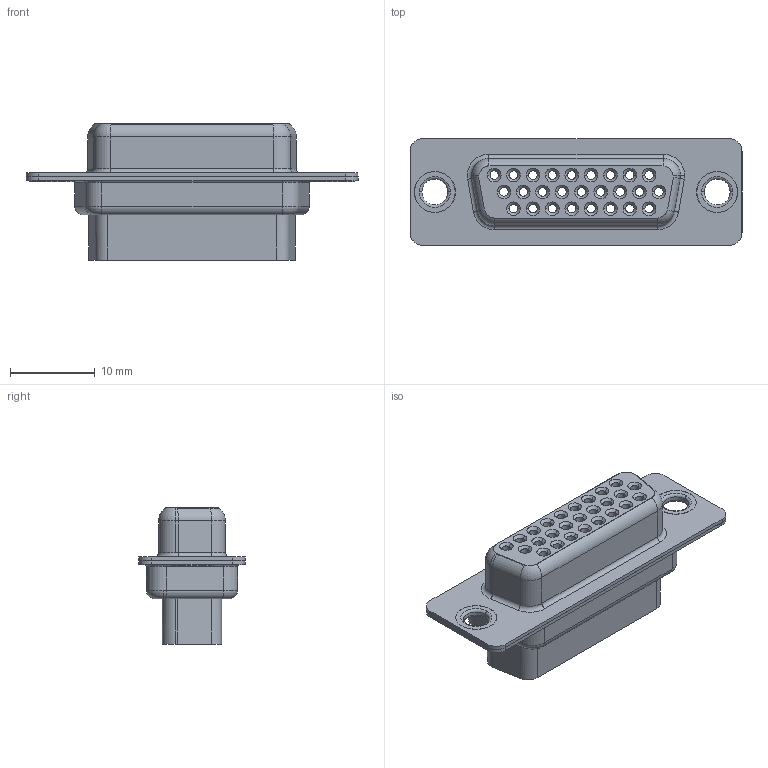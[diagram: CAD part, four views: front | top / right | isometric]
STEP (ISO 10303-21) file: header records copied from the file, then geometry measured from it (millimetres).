
FILE_DESCRIPTION (( 'STEP AP203' ), '1' );
FILE_NAME ('638-026-010-041.STEP', '2020-07-18T16:34:46', ( '' ), ( '' ), 'SwSTEP 2.0', 'SolidWorks 2020', '' );
FILE_SCHEMA (( 'CONFIG_CONTROL_DESIGN' ));
Length unit declared in the file: millimetre
Products named in the file (5): 638-026-010-041; 638 Shell Rear_26 Contacts; 638 Housing_26 Contacts HP; 638 Shell Front_26 Contacts; 638 Thru Hole Rivet
Assembly tree (5 placements, depth 2):
  638-026-010-041
    638 Housing_26 Contacts HP
    638 Shell Front_26 Contacts
    638 Shell Rear_26 Contacts
    638 Thru Hole Rivet  x2
Bounding box: 39.19 x 12.6 x 16.1 mm (x, y, z)
Volume: 2299.5 mm3; surface area: 6292.6 mm2
Topology: 5 solids, 5 shells, 591 faces, 1331 edges, 839 vertices
Faces by surface type: cylinder 329, plane 145, torus 65, cone 52
Entity records: 16962 total; most frequent: DIRECTION 3155, CARTESIAN_POINT 2870, ORIENTED_EDGE 2582, AXIS2_PLACEMENT_3D 1330, EDGE_CURVE 1291, VERTEX_POINT 815, CIRCLE 751, EDGE_LOOP 724
